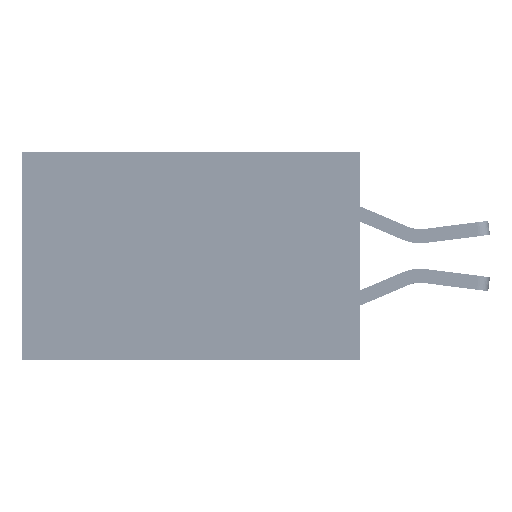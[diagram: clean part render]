
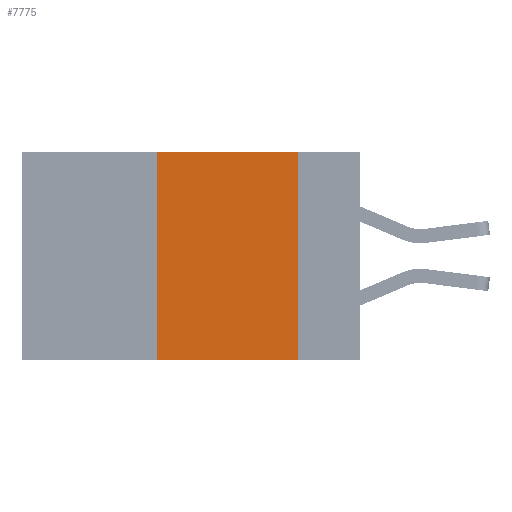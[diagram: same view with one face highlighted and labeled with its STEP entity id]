
A CAD part, left-side view. The second image highlights one B-rep face of the part: STEP entity #7775.
In plain terms, the highlighted planar face has unit normal (-1, 0, 0).
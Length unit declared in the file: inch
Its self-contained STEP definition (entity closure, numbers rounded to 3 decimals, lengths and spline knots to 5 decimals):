
#627 = CARTESIAN_POINT ( 'NONE',  ( 0., 0.11, 0. ) ) ;
#1454 = CARTESIAN_POINT ( 'NONE',  ( 0., 0.36, 0. ) ) ;
#3591 = CARTESIAN_POINT ( 'NONE',  ( 0., 0.36, 0. ) ) ;
#6289 = ORIENTED_EDGE ( 'NONE', *, *, #8768, .F. ) ;
#7775 = ADVANCED_FACE ( 'NONE', ( #11354 ), #16573, .F. ) ;
#8604 = DIRECTION ( 'NONE',  ( 0., 0., -1. ) ) ;
#8768 = EDGE_CURVE ( 'NONE', #29420, #11526, #10651, .T. ) ;
#10222 = CARTESIAN_POINT ( 'NONE',  ( 0., 0.6, 0. ) ) ;
#10651 = LINE ( 'NONE', #10222, #26766 ) ;
#11354 = FACE_OUTER_BOUND ( 'NONE', #38576, .T. ) ;
#11526 = VERTEX_POINT ( 'NONE', #627 ) ;
#12430 = EDGE_CURVE ( 'NONE', #20807, #40683, #30465, .T. ) ;
#13253 = DIRECTION ( 'NONE',  ( 0., 0., -1. ) ) ;
#14572 = EDGE_CURVE ( 'NONE', #11526, #40683, #33254, .T. ) ;
#16573 = PLANE ( 'NONE',  #39722 ) ;
#18774 = CARTESIAN_POINT ( 'NONE',  ( 0., 0.11, 0. ) ) ;
#19275 = VECTOR ( 'NONE', #8604, 39.37008 ) ;
#20505 = ORIENTED_EDGE ( 'NONE', *, *, #14572, .F. ) ;
#20807 = VERTEX_POINT ( 'NONE', #40755 ) ;
#24337 = EDGE_CURVE ( 'NONE', #20807, #29420, #33669, .T. ) ;
#25846 = ORIENTED_EDGE ( 'NONE', *, *, #24337, .F. ) ;
#26766 = VECTOR ( 'NONE', #27296, 39.37008 ) ;
#27296 = DIRECTION ( 'NONE',  ( 0., -1., 0. ) ) ;
#28867 = DIRECTION ( 'NONE',  ( 0., 0., 1. ) ) ;
#29420 = VERTEX_POINT ( 'NONE', #3591 ) ;
#30465 = LINE ( 'NONE', #32759, #34225 ) ;
#32759 = CARTESIAN_POINT ( 'NONE',  ( 0., 0.6, -0.37 ) ) ;
#33254 = LINE ( 'NONE', #18774, #19275 ) ;
#33669 = LINE ( 'NONE', #1454, #42217 ) ;
#33882 = CARTESIAN_POINT ( 'NONE',  ( 0., 0.6, 0. ) ) ;
#34225 = VECTOR ( 'NONE', #39783, 39.37008 ) ;
#38576 = EDGE_LOOP ( 'NONE', ( #20505, #6289, #25846, #41641 ) ) ;
#39722 = AXIS2_PLACEMENT_3D ( 'NONE', #33882, #43621, #13253 ) ;
#39783 = DIRECTION ( 'NONE',  ( 0., -1., 0. ) ) ;
#40683 = VERTEX_POINT ( 'NONE', #42713 ) ;
#40755 = CARTESIAN_POINT ( 'NONE',  ( 0., 0.36, -0.37 ) ) ;
#41641 = ORIENTED_EDGE ( 'NONE', *, *, #12430, .T. ) ;
#42217 = VECTOR ( 'NONE', #28867, 39.37008 ) ;
#42713 = CARTESIAN_POINT ( 'NONE',  ( 0., 0.11, -0.37 ) ) ;
#43621 = DIRECTION ( 'NONE',  ( 1., 0., 0. ) ) ;
